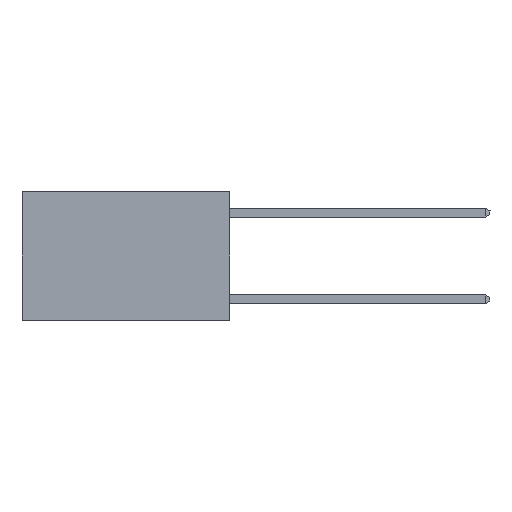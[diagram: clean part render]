
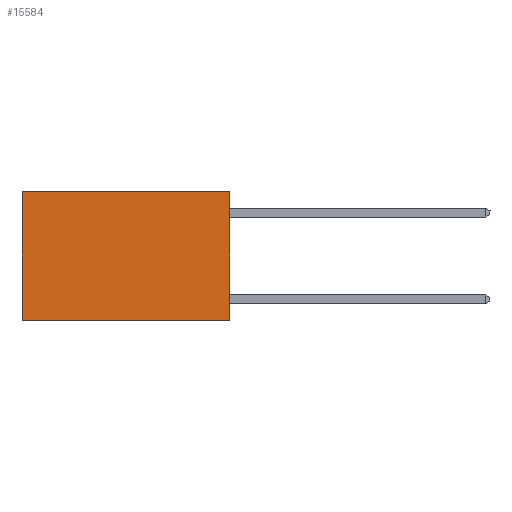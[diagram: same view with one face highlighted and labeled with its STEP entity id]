
A CAD part, left-side view. The second image highlights one B-rep face of the part: STEP entity #15584.
In plain terms, the highlighted planar face has unit normal (-1, 0, 0).
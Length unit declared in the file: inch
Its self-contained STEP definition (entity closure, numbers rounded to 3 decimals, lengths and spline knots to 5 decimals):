
#959 = ORIENTED_EDGE ( 'NONE', *, *, #18169, .T. ) ;
#1191 = DIRECTION ( 'NONE',  ( 0., 0., -1. ) ) ;
#1413 = LINE ( 'NONE', #16161, #23095 ) ;
#1673 = CARTESIAN_POINT ( 'NONE',  ( 0.2625, 0.6, -0.37 ) ) ;
#3273 = LINE ( 'NONE', #22777, #23473 ) ;
#3513 = CARTESIAN_POINT ( 'NONE',  ( 0.2625, 0., 0. ) ) ;
#4559 = VECTOR ( 'NONE', #14359, 39.37008 ) ;
#4682 = CARTESIAN_POINT ( 'NONE',  ( 0.2625, 0., 0. ) ) ;
#6080 = ORIENTED_EDGE ( 'NONE', *, *, #7506, .F. ) ;
#6336 = FACE_OUTER_BOUND ( 'NONE', #7245, .T. ) ;
#7052 = ORIENTED_EDGE ( 'NONE', *, *, #7679, .F. ) ;
#7245 = EDGE_LOOP ( 'NONE', ( #19305, #7052, #6080, #959 ) ) ;
#7502 = DIRECTION ( 'NONE',  ( 0., 1., 0. ) ) ;
#7506 = EDGE_CURVE ( 'NONE', #12308, #10991, #13144, .T. ) ;
#7559 = AXIS2_PLACEMENT_3D ( 'NONE', #8825, #16470, #22440 ) ;
#7679 = EDGE_CURVE ( 'NONE', #10991, #22887, #21766, .T. ) ;
#8825 = CARTESIAN_POINT ( 'NONE',  ( 0.2625, 0., 0. ) ) ;
#10603 = EDGE_CURVE ( 'NONE', #10798, #22887, #1413, .T. ) ;
#10798 = VERTEX_POINT ( 'NONE', #11227 ) ;
#10807 = PLANE ( 'NONE',  #7559 ) ;
#10991 = VERTEX_POINT ( 'NONE', #13696 ) ;
#11227 = CARTESIAN_POINT ( 'NONE',  ( 0.2625, 0.6, 0. ) ) ;
#12303 = CARTESIAN_POINT ( 'NONE',  ( 0.2625, 0., -0.37 ) ) ;
#12308 = VERTEX_POINT ( 'NONE', #4682 ) ;
#13144 = LINE ( 'NONE', #3513, #23545 ) ;
#13696 = CARTESIAN_POINT ( 'NONE',  ( 0.2625, 0., -0.37 ) ) ;
#14359 = DIRECTION ( 'NONE',  ( 0., 1., 0. ) ) ;
#15584 = ADVANCED_FACE ( 'NONE', ( #6336 ), #10807, .F. ) ;
#16161 = CARTESIAN_POINT ( 'NONE',  ( 0.2625, 0.6, 0. ) ) ;
#16470 = DIRECTION ( 'NONE',  ( 1., 0., 0. ) ) ;
#18169 = EDGE_CURVE ( 'NONE', #12308, #10798, #3273, .T. ) ;
#19305 = ORIENTED_EDGE ( 'NONE', *, *, #10603, .T. ) ;
#21766 = LINE ( 'NONE', #12303, #4559 ) ;
#22440 = DIRECTION ( 'NONE',  ( 0., 0., -1. ) ) ;
#22611 = DIRECTION ( 'NONE',  ( 0., 0., -1. ) ) ;
#22777 = CARTESIAN_POINT ( 'NONE',  ( 0.2625, 0., 0. ) ) ;
#22887 = VERTEX_POINT ( 'NONE', #1673 ) ;
#23095 = VECTOR ( 'NONE', #1191, 39.37008 ) ;
#23473 = VECTOR ( 'NONE', #7502, 39.37008 ) ;
#23545 = VECTOR ( 'NONE', #22611, 39.37008 ) ;
